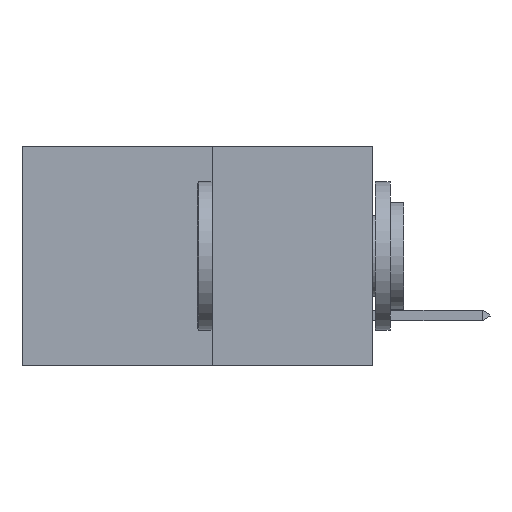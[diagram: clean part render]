
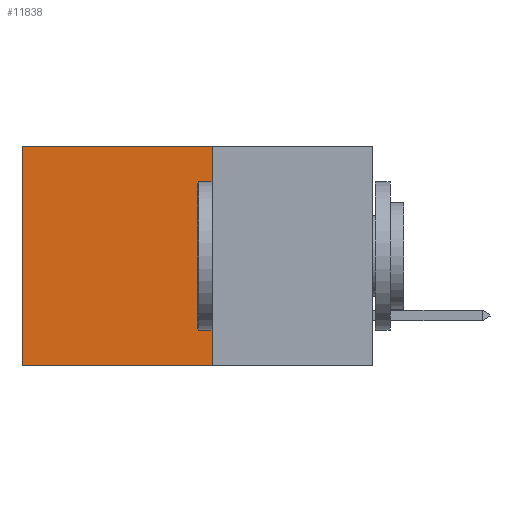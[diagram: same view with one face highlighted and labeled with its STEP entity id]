
A CAD part, left-side view. The second image highlights one B-rep face of the part: STEP entity #11838.
In plain terms, the highlighted planar face has unit normal (-1, 0, 0).
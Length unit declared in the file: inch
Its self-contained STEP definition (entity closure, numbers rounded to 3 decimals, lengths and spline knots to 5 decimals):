
#948 = DIRECTION ( 'NONE',  ( 0., 0., -1. ) ) ;
#1042 = VECTOR ( 'NONE', #12415, 39.37008 ) ;
#1055 = CARTESIAN_POINT ( 'NONE',  ( 0.277, 0.27, -0.37 ) ) ;
#1173 = DIRECTION ( 'NONE',  ( 0., 0., -1. ) ) ;
#2144 = VERTEX_POINT ( 'NONE', #11825 ) ;
#3711 = CARTESIAN_POINT ( 'NONE',  ( 0.277, 0.59, -0.37 ) ) ;
#3963 = VECTOR ( 'NONE', #14270, 39.37008 ) ;
#4513 = VECTOR ( 'NONE', #948, 39.37008 ) ;
#4780 = LINE ( 'NONE', #11121, #1042 ) ;
#4908 = AXIS2_PLACEMENT_3D ( 'NONE', #14732, #7018, #16025 ) ;
#5669 = PLANE ( 'NONE',  #4908 ) ;
#7018 = DIRECTION ( 'NONE',  ( 1., 0., 0. ) ) ;
#7382 = EDGE_LOOP ( 'NONE', ( #15022, #16531, #16494, #15684 ) ) ;
#7480 = EDGE_CURVE ( 'NONE', #2144, #8585, #14304, .T. ) ;
#7576 = LINE ( 'NONE', #10382, #3963 ) ;
#7686 = FACE_OUTER_BOUND ( 'NONE', #7382, .T. ) ;
#7836 = VECTOR ( 'NONE', #1173, 39.37008 ) ;
#8585 = VERTEX_POINT ( 'NONE', #14882 ) ;
#8910 = EDGE_CURVE ( 'NONE', #2144, #9016, #7576, .T. ) ;
#8918 = LINE ( 'NONE', #9118, #4513 ) ;
#9016 = VERTEX_POINT ( 'NONE', #15771 ) ;
#9118 = CARTESIAN_POINT ( 'NONE',  ( 0.277, 0.59, -0.37 ) ) ;
#10382 = CARTESIAN_POINT ( 'NONE',  ( 0.277, 0.27, 0. ) ) ;
#10572 = EDGE_CURVE ( 'NONE', #8585, #15151, #4780, .T. ) ;
#11121 = CARTESIAN_POINT ( 'NONE',  ( 0.277, 0.27, -0.37 ) ) ;
#11825 = CARTESIAN_POINT ( 'NONE',  ( 0.277, 0.27, 0. ) ) ;
#11838 = ADVANCED_FACE ( 'NONE', ( #7686 ), #5669, .F. ) ;
#12189 = EDGE_CURVE ( 'NONE', #9016, #15151, #8918, .T. ) ;
#12415 = DIRECTION ( 'NONE',  ( 0., 1., 0. ) ) ;
#14270 = DIRECTION ( 'NONE',  ( 0., 1., 0. ) ) ;
#14304 = LINE ( 'NONE', #1055, #7836 ) ;
#14732 = CARTESIAN_POINT ( 'NONE',  ( 0.277, 0.27, -0.37 ) ) ;
#14882 = CARTESIAN_POINT ( 'NONE',  ( 0.277, 0.27, -0.37 ) ) ;
#15022 = ORIENTED_EDGE ( 'NONE', *, *, #12189, .T. ) ;
#15151 = VERTEX_POINT ( 'NONE', #3711 ) ;
#15684 = ORIENTED_EDGE ( 'NONE', *, *, #8910, .T. ) ;
#15771 = CARTESIAN_POINT ( 'NONE',  ( 0.277, 0.59, 0. ) ) ;
#16025 = DIRECTION ( 'NONE',  ( 0., 0., -1. ) ) ;
#16494 = ORIENTED_EDGE ( 'NONE', *, *, #7480, .F. ) ;
#16531 = ORIENTED_EDGE ( 'NONE', *, *, #10572, .F. ) ;
